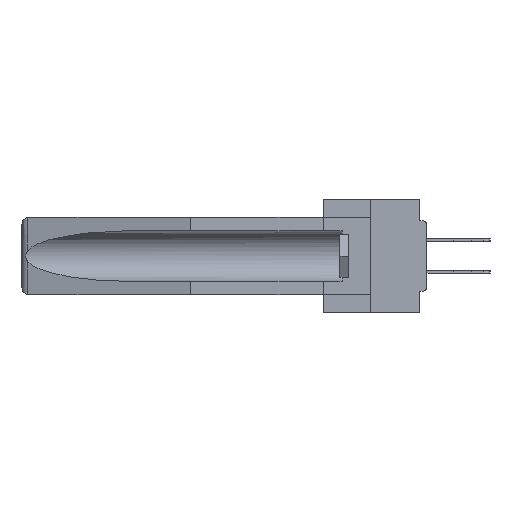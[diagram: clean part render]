
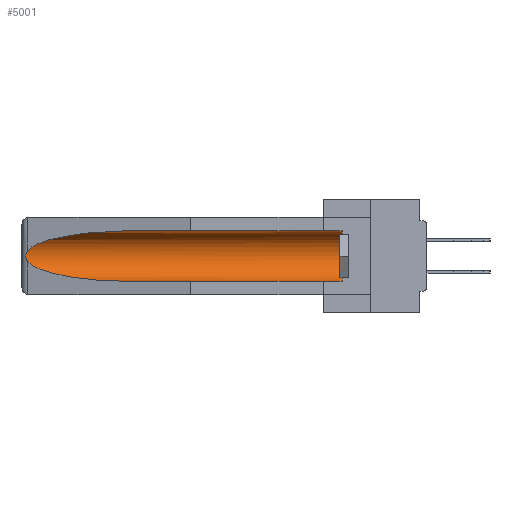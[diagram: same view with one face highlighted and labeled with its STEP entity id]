
A CAD part, left-side view. The second image highlights one B-rep face of the part: STEP entity #5001.
In plain terms, the highlighted cylindrical face has radius 2.857 mm (diameter 5.715 mm), a partial arc.
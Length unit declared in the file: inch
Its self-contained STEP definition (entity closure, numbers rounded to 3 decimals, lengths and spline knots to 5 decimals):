
#1704 = VERTEX_POINT ( 'NONE', #28593 ) ;
#2492 = CARTESIAN_POINT ( 'NONE',  ( 0.155, -0.30754, -0.284 ) ) ;
#2773 = ORIENTED_EDGE ( 'NONE', *, *, #11955, .T. ) ;
#2831 = CARTESIAN_POINT ( 'NONE',  ( 0.155, 1.07973, -0.059 ) ) ;
#2973 = CYLINDRICAL_SURFACE ( 'NONE', #11970, 0.1125 ) ;
#4291 = VERTEX_POINT ( 'NONE', #8129 ) ;
#4944 = CARTESIAN_POINT ( 'NONE',  ( 0.26537, 1.52718, -0.14972 ) ) ;
#5001 = ADVANCED_FACE ( 'NONE', ( #28817 ), #2973, .F. ) ;
#6368 = CARTESIAN_POINT ( 'NONE',  ( 0.155, 0.126, -0.1715 ) ) ;
#6862 = ORIENTED_EDGE ( 'NONE', *, *, #35041, .T. ) ;
#8129 = CARTESIAN_POINT ( 'NONE',  ( 0.155, 0.126, -0.284 ) ) ;
#8394 = ORIENTED_EDGE ( 'NONE', *, *, #25643, .T. ) ;
#8414 = EDGE_CURVE ( 'NONE', #4291, #22797, #34498, .T. ) ;
#8447 = DIRECTION ( 'NONE',  ( 0., 1., 0. ) ) ;
#9353 = EDGE_LOOP ( 'NONE', ( #2773, #8394, #6862, #19681, #23377, #22266 ) ) ;
#9597 = DIRECTION ( 'NONE',  ( 0., 0., 1. ) ) ;
#10523 = CARTESIAN_POINT ( 'NONE',  ( 0.155, 1.07973, -0.284 ) ) ;
#11281 =( BOUNDED_CURVE ( )  B_SPLINE_CURVE ( 3, ( #2831, #32307, #32181, #35367 ),
 .UNSPECIFIED., .F., .F. ) 
 B_SPLINE_CURVE_WITH_KNOTS ( ( 4, 4 ),
 ( 4.71239, 6.08839 ),
 .UNSPECIFIED. ) 
 CURVE ( )  GEOMETRIC_REPRESENTATION_ITEM ( )  RATIONAL_B_SPLINE_CURVE ( ( 1., 0.848, 0.848, 1. ) ) 
 REPRESENTATION_ITEM ( '' )  );
#11504 = DIRECTION ( 'NONE',  ( 0., 1., 0. ) ) ;
#11747 = CARTESIAN_POINT ( 'NONE',  ( 0.26537, 1.52718, -0.19328 ) ) ;
#11955 = EDGE_CURVE ( 'NONE', #1704, #22030, #11281, .T. ) ;
#11970 = AXIS2_PLACEMENT_3D ( 'NONE', #31096, #8447, #37211 ) ;
#12333 = VECTOR ( 'NONE', #11504, 39.37008 ) ;
#12509 = EDGE_CURVE ( 'NONE', #22797, #1704, #36690, .T. ) ;
#14380 = CARTESIAN_POINT ( 'NONE',  ( 0.26597, 1.52961, -0.15275 ) ) ;
#15830 = DIRECTION ( 'NONE',  ( 0., 1., 0. ) ) ;
#17978 = CARTESIAN_POINT ( 'NONE',  ( 0.26537, 1.52718, -0.14972 ) ) ;
#18257 = VECTOR ( 'NONE', #15830, 39.37008 ) ;
#19681 = ORIENTED_EDGE ( 'NONE', *, *, #20724, .F. ) ;
#20724 = EDGE_CURVE ( 'NONE', #4291, #33028, #26714, .T. ) ;
#20727 = CARTESIAN_POINT ( 'NONE',  ( 0.2673, 1.5327, -0.16383 ) ) ;
#22030 = VERTEX_POINT ( 'NONE', #4944 ) ;
#22266 = ORIENTED_EDGE ( 'NONE', *, *, #12509, .T. ) ;
#22797 = VERTEX_POINT ( 'NONE', #31357 ) ;
#23204 = AXIS2_PLACEMENT_3D ( 'NONE', #6368, #35030, #9597 ) ;
#23377 = ORIENTED_EDGE ( 'NONE', *, *, #8414, .T. ) ;
#23964 = CARTESIAN_POINT ( 'NONE',  ( 0.26654, 1.53092, -0.15636 ) ) ;
#23976 = CARTESIAN_POINT ( 'NONE',  ( 0.26537, 1.52718, -0.19328 ) ) ;
#25643 = EDGE_CURVE ( 'NONE', #22030, #37814, #37234, .T. ) ;
#26325 = CARTESIAN_POINT ( 'NONE',  ( 0.21114, 1.30732, -0.284 ) ) ;
#26714 = LINE ( 'NONE', #2492, #18257 ) ;
#27296 = CARTESIAN_POINT ( 'NONE',  ( 0.26597, 1.5296, -0.19026 ) ) ;
#27304 =( BOUNDED_CURVE ( )  B_SPLINE_CURVE ( 3, ( #28832, #32217, #26325, #10523 ),
 .UNSPECIFIED., .F., .F. ) 
 B_SPLINE_CURVE_WITH_KNOTS ( ( 4, 4 ),
 ( 0.1948, 1.5708 ),
 .UNSPECIFIED. ) 
 CURVE ( )  GEOMETRIC_REPRESENTATION_ITEM ( )  RATIONAL_B_SPLINE_CURVE ( ( 1., 0.848, 0.848, 1. ) ) 
 REPRESENTATION_ITEM ( '' )  );
#28593 = CARTESIAN_POINT ( 'NONE',  ( 0.155, 1.07973, -0.059 ) ) ;
#28817 = FACE_OUTER_BOUND ( 'NONE', #9353, .T. ) ;
#28832 = CARTESIAN_POINT ( 'NONE',  ( 0.26537, 1.52718, -0.19328 ) ) ;
#31096 = CARTESIAN_POINT ( 'NONE',  ( 0.155, -0.30754, -0.1715 ) ) ;
#31357 = CARTESIAN_POINT ( 'NONE',  ( 0.155, 0.126, -0.059 ) ) ;
#32181 = CARTESIAN_POINT ( 'NONE',  ( 0.25451, 1.48313, -0.09465 ) ) ;
#32217 = CARTESIAN_POINT ( 'NONE',  ( 0.25451, 1.48313, -0.24835 ) ) ;
#32307 = CARTESIAN_POINT ( 'NONE',  ( 0.21114, 1.30732, -0.059 ) ) ;
#33028 = VERTEX_POINT ( 'NONE', #40246 ) ;
#33432 = CARTESIAN_POINT ( 'NONE',  ( 0.2675, 1.53308, -0.17534 ) ) ;
#33980 = CARTESIAN_POINT ( 'NONE',  ( 0.2675, 1.53308, -0.16763 ) ) ;
#34498 = CIRCLE ( 'NONE', #23204, 0.1125 ) ;
#35030 = DIRECTION ( 'NONE',  ( 0., -1., 0. ) ) ;
#35041 = EDGE_CURVE ( 'NONE', #37814, #33028, #27304, .T. ) ;
#35367 = CARTESIAN_POINT ( 'NONE',  ( 0.26537, 1.52718, -0.14972 ) ) ;
#36626 = CARTESIAN_POINT ( 'NONE',  ( 0.26655, 1.53094, -0.18657 ) ) ;
#36690 = LINE ( 'NONE', #37186, #12333 ) ;
#36764 = CARTESIAN_POINT ( 'NONE',  ( 0.2673, 1.53269, -0.17917 ) ) ;
#37186 = CARTESIAN_POINT ( 'NONE',  ( 0.155, -0.30754, -0.059 ) ) ;
#37211 = DIRECTION ( 'NONE',  ( 0., 0., 1. ) ) ;
#37234 = B_SPLINE_CURVE_WITH_KNOTS ( 'NONE', 3,
 ( #17978, #14380, #23964, #20727, #33980, #33432, #36764, #36626, #27296, #11747 ),
 .UNSPECIFIED., .F., .F.,
 ( 4, 2, 2, 2, 4 ),
 ( 0., 0.00029, 0.00058, 0.00087, 0.00117 ),
 .UNSPECIFIED. ) ;
#37814 = VERTEX_POINT ( 'NONE', #23976 ) ;
#40246 = CARTESIAN_POINT ( 'NONE',  ( 0.155, 1.07973, -0.284 ) ) ;
